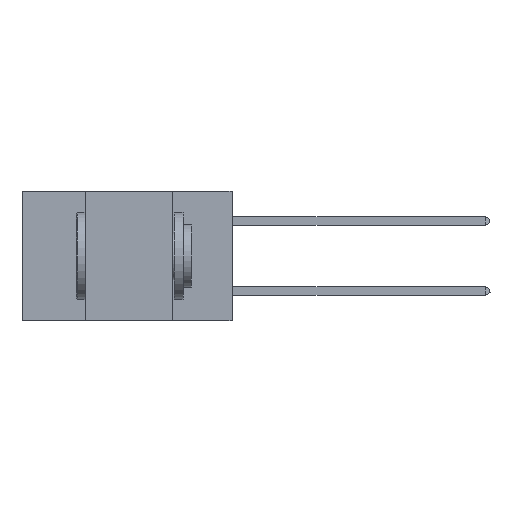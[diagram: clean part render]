
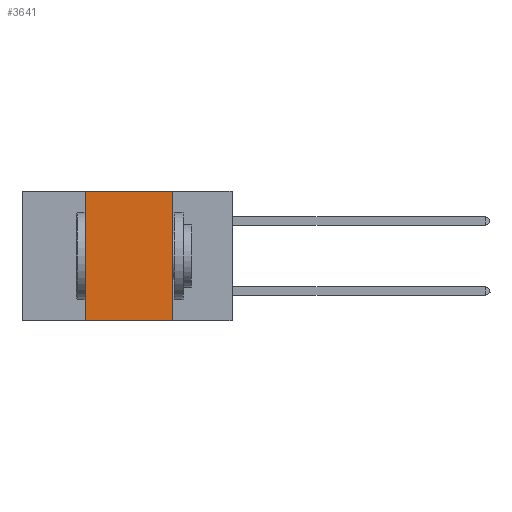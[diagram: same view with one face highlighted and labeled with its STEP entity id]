
A CAD part, left-side view. The second image highlights one B-rep face of the part: STEP entity #3641.
In plain terms, the highlighted planar face has unit normal (-1, 0, 0).
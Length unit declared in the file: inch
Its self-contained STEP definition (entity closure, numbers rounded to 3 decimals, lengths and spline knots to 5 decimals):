
#163 = EDGE_CURVE ( 'NONE', #12270, #7480, #13488, .T. ) ;
#370 = CARTESIAN_POINT ( 'NONE',  ( 0., 0.17, 0. ) ) ;
#801 = VECTOR ( 'NONE', #8285, 39.37008 ) ;
#1268 = ORIENTED_EDGE ( 'NONE', *, *, #10170, .T. ) ;
#1383 = DIRECTION ( 'NONE',  ( 0., -1., 0. ) ) ;
#1735 = ORIENTED_EDGE ( 'NONE', *, *, #13993, .F. ) ;
#2795 = EDGE_CURVE ( 'NONE', #6034, #8166, #14043, .T. ) ;
#3124 = PLANE ( 'NONE',  #15623 ) ;
#3415 = DIRECTION ( 'NONE',  ( 1., 0., 0. ) ) ;
#3641 = ADVANCED_FACE ( 'NONE', ( #13447 ), #3124, .F. ) ;
#4443 = CARTESIAN_POINT ( 'NONE',  ( 0., 0.17, 0. ) ) ;
#5690 = CARTESIAN_POINT ( 'NONE',  ( 0., 0.42, 0. ) ) ;
#6034 = VERTEX_POINT ( 'NONE', #10388 ) ;
#7234 = VECTOR ( 'NONE', #1383, 39.37008 ) ;
#7480 = VERTEX_POINT ( 'NONE', #15240 ) ;
#8166 = VERTEX_POINT ( 'NONE', #15275 ) ;
#8228 = DIRECTION ( 'NONE',  ( 0., -1., 0. ) ) ;
#8285 = DIRECTION ( 'NONE',  ( 0., 0., 1. ) ) ;
#9079 = LINE ( 'NONE', #9248, #7234 ) ;
#9248 = CARTESIAN_POINT ( 'NONE',  ( 0., 0.6, 0. ) ) ;
#9740 = LINE ( 'NONE', #10513, #10765 ) ;
#10170 = EDGE_CURVE ( 'NONE', #6034, #7480, #9740, .T. ) ;
#10388 = CARTESIAN_POINT ( 'NONE',  ( 0., 0.42, -0.37 ) ) ;
#10513 = CARTESIAN_POINT ( 'NONE',  ( 0., 0.6, -0.37 ) ) ;
#10765 = VECTOR ( 'NONE', #8228, 39.37008 ) ;
#11528 = ORIENTED_EDGE ( 'NONE', *, *, #2795, .F. ) ;
#12270 = VERTEX_POINT ( 'NONE', #4443 ) ;
#12496 = DIRECTION ( 'NONE',  ( 0., 0., -1. ) ) ;
#13447 = FACE_OUTER_BOUND ( 'NONE', #13847, .T. ) ;
#13488 = LINE ( 'NONE', #370, #16333 ) ;
#13847 = EDGE_LOOP ( 'NONE', ( #14049, #1735, #11528, #1268 ) ) ;
#13972 = DIRECTION ( 'NONE',  ( 0., 0., -1. ) ) ;
#13993 = EDGE_CURVE ( 'NONE', #8166, #12270, #9079, .T. ) ;
#14043 = LINE ( 'NONE', #5690, #801 ) ;
#14049 = ORIENTED_EDGE ( 'NONE', *, *, #163, .F. ) ;
#14838 = CARTESIAN_POINT ( 'NONE',  ( 0., 0.6, 0. ) ) ;
#15240 = CARTESIAN_POINT ( 'NONE',  ( 0., 0.17, -0.37 ) ) ;
#15275 = CARTESIAN_POINT ( 'NONE',  ( 0., 0.42, 0. ) ) ;
#15623 = AXIS2_PLACEMENT_3D ( 'NONE', #14838, #3415, #12496 ) ;
#16333 = VECTOR ( 'NONE', #13972, 39.37008 ) ;
